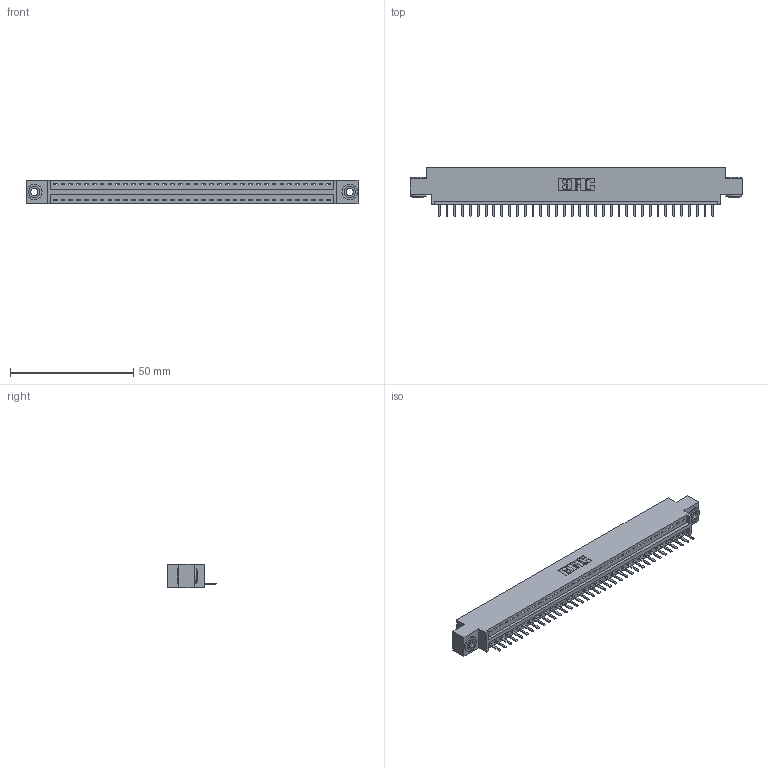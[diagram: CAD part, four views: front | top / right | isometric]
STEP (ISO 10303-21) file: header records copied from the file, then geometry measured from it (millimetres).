
FILE_DESCRIPTION (( 'STEP AP203' ), '1' );
FILE_NAME ('396-036-520-603.STEP', '2018-09-06T03:20:03', ( '' ), ( '' ), 'SwSTEP 2.0', 'SolidWorks 2016', '' );
FILE_SCHEMA (( 'CONFIG_CONTROL_DESIGN' ));
Length unit declared in the file: inch
Products named in the file (4): 346 Part_0.170 Offset - 0.156 Dia-TH; 345-292-001_345-293-120; 345-250-002_345-250-002-102; 396-036-520-603
Assembly tree (39 placements, depth 2):
  396-036-520-603
    346 Part_0.170 Offset - 0.156 Dia-TH
    345-292-001_345-293-120  x36
    345-250-002_345-250-002-102  x2
Bounding box: 134.87 x 20.02 x 9.4 mm (x, y, z)
Volume: 12630.3 mm3; surface area: 15755.4 mm2
Topology: 39 solids, 39 shells, 2396 faces, 7041 edges, 4594 vertices
Faces by surface type: plane 1602, cylinder 786, cone 8
Entity records: 24046 total; most frequent: CARTESIAN_POINT 4115, ORIENTED_EDGE 4066, DIRECTION 3655, EDGE_CURVE 2033, LINE 1729, VECTOR 1729, VERTEX_POINT 1350, AXIS2_PLACEMENT_3D 963
